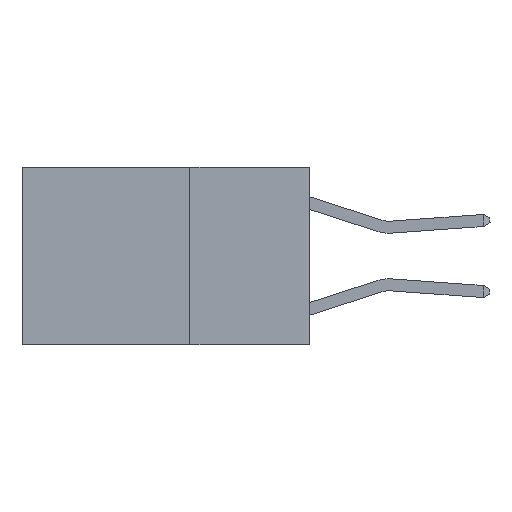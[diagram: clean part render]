
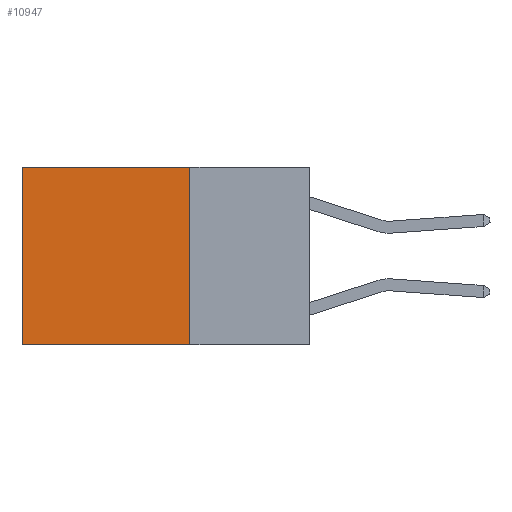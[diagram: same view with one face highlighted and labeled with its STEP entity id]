
A CAD part, left-side view. The second image highlights one B-rep face of the part: STEP entity #10947.
In plain terms, the highlighted planar face has unit normal (-1, 0, 0).
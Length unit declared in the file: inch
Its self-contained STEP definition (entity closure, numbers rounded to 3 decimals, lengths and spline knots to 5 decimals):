
#104 = DIRECTION ( 'NONE',  ( 0., 0., -1. ) ) ;
#1220 = VECTOR ( 'NONE', #104, 39.37008 ) ;
#2243 = VERTEX_POINT ( 'NONE', #17201 ) ;
#2632 = EDGE_LOOP ( 'NONE', ( #3298, #3355, #3457, #3607 ) ) ;
#2704 = FACE_OUTER_BOUND ( 'NONE', #2632, .T. ) ;
#3228 = CARTESIAN_POINT ( 'NONE',  ( 0.2625, 0.25, 0. ) ) ;
#3298 = ORIENTED_EDGE ( 'NONE', *, *, #18735, .T. ) ;
#3355 = ORIENTED_EDGE ( 'NONE', *, *, #10093, .F. ) ;
#3457 = ORIENTED_EDGE ( 'NONE', *, *, #7187, .F. ) ;
#3607 = ORIENTED_EDGE ( 'NONE', *, *, #12306, .T. ) ;
#4341 = DIRECTION ( 'NONE',  ( 0., 0., -1. ) ) ;
#4411 = CARTESIAN_POINT ( 'NONE',  ( 0.2625, 0.25, 0. ) ) ;
#4587 = VECTOR ( 'NONE', #13523, 39.37008 ) ;
#5230 = CARTESIAN_POINT ( 'NONE',  ( 0.2625, 0.6, 0. ) ) ;
#5921 = VECTOR ( 'NONE', #15202, 39.37008 ) ;
#6058 = CARTESIAN_POINT ( 'NONE',  ( 0.2625, 0.25, 0. ) ) ;
#6918 = CARTESIAN_POINT ( 'NONE',  ( 0.2625, 0.25, -0.37 ) ) ;
#7187 = EDGE_CURVE ( 'NONE', #10980, #13255, #13894, .T. ) ;
#8825 = LINE ( 'NONE', #6918, #16321 ) ;
#9939 = DIRECTION ( 'NONE',  ( 0., 1., 0. ) ) ;
#10093 = EDGE_CURVE ( 'NONE', #13255, #2243, #8825, .T. ) ;
#10947 = ADVANCED_FACE ( 'NONE', ( #2704 ), #13267, .F. ) ;
#10980 = VERTEX_POINT ( 'NONE', #4411 ) ;
#12306 = EDGE_CURVE ( 'NONE', #10980, #17467, #12578, .T. ) ;
#12578 = LINE ( 'NONE', #6058, #4587 ) ;
#12862 = AXIS2_PLACEMENT_3D ( 'NONE', #19113, #13326, #4341 ) ;
#13236 = LINE ( 'NONE', #18106, #1220 ) ;
#13255 = VERTEX_POINT ( 'NONE', #14073 ) ;
#13267 = PLANE ( 'NONE',  #12862 ) ;
#13326 = DIRECTION ( 'NONE',  ( 1., 0., 0. ) ) ;
#13523 = DIRECTION ( 'NONE',  ( 0., 1., 0. ) ) ;
#13894 = LINE ( 'NONE', #3228, #5921 ) ;
#14073 = CARTESIAN_POINT ( 'NONE',  ( 0.2625, 0.25, -0.37 ) ) ;
#15202 = DIRECTION ( 'NONE',  ( 0., 0., -1. ) ) ;
#16321 = VECTOR ( 'NONE', #9939, 39.37008 ) ;
#17201 = CARTESIAN_POINT ( 'NONE',  ( 0.2625, 0.6, -0.37 ) ) ;
#17467 = VERTEX_POINT ( 'NONE', #5230 ) ;
#18106 = CARTESIAN_POINT ( 'NONE',  ( 0.2625, 0.6, 0. ) ) ;
#18735 = EDGE_CURVE ( 'NONE', #17467, #2243, #13236, .T. ) ;
#19113 = CARTESIAN_POINT ( 'NONE',  ( 0.2625, 0.25, 0. ) ) ;
